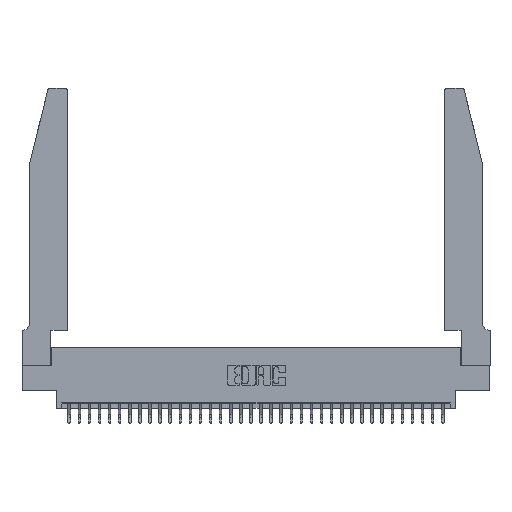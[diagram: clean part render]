
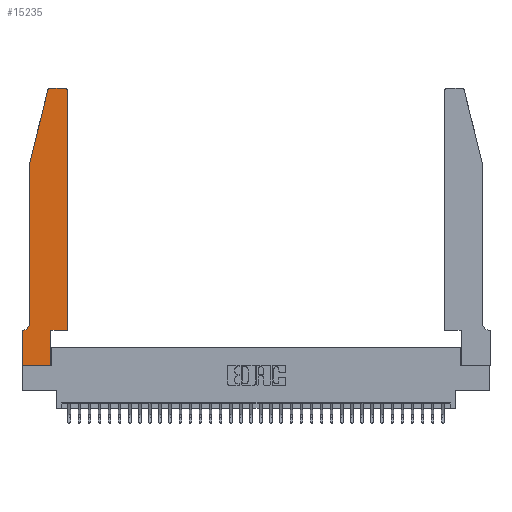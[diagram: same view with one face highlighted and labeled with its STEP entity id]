
A CAD part, top view. The second image highlights one B-rep face of the part: STEP entity #15235.
In plain terms, the highlighted planar face has unit normal (0, 0, 1).
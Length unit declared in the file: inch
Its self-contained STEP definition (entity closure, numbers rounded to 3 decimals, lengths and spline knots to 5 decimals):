
#98 = LINE ( 'NONE', #8439, #7492 ) ;
#121 = VECTOR ( 'NONE', #23977, 39.37008 ) ;
#1457 = CARTESIAN_POINT ( 'NONE',  ( 0.2865, 0.35, 0.37 ) ) ;
#1524 = AXIS2_PLACEMENT_3D ( 'NONE', #26962, #10634, #29683 ) ;
#1671 = VECTOR ( 'NONE', #10554, 39.37008 ) ;
#1958 = DIRECTION ( 'NONE',  ( 1., 0., 0. ) ) ;
#2000 = CARTESIAN_POINT ( 'NONE',  ( 0.0755, 2., 0.37 ) ) ;
#2250 = CARTESIAN_POINT ( 'NONE',  ( 0.0755, 2., 0.37 ) ) ;
#2755 = EDGE_CURVE ( 'NONE', #16288, #17330, #23582, .T. ) ;
#3211 = VECTOR ( 'NONE', #24135, 39.37008 ) ;
#3431 = EDGE_CURVE ( 'NONE', #17330, #6809, #3760, .T. ) ;
#3760 = CIRCLE ( 'NONE', #1524, 0.03 ) ;
#4895 = CARTESIAN_POINT ( 'NONE',  ( 0., 0., 0.37 ) ) ;
#5574 = EDGE_CURVE ( 'NONE', #13917, #17988, #11427, .T. ) ;
#5582 = ORIENTED_EDGE ( 'NONE', *, *, #17892, .T. ) ;
#5916 = AXIS2_PLACEMENT_3D ( 'NONE', #6968, #26132, #9776 ) ;
#6114 = VERTEX_POINT ( 'NONE', #1457 ) ;
#6215 = CARTESIAN_POINT ( 'NONE',  ( 0.2865, 0., 0.37 ) ) ;
#6584 = VECTOR ( 'NONE', #7798, 39.37008 ) ;
#6809 = VERTEX_POINT ( 'NONE', #15743 ) ;
#6968 = CARTESIAN_POINT ( 'NONE',  ( 0., 0.35, 0.37 ) ) ;
#7492 = VECTOR ( 'NONE', #16575, 39.37008 ) ;
#7798 = DIRECTION ( 'NONE',  ( 0., 1., 0. ) ) ;
#8439 = CARTESIAN_POINT ( 'NONE',  ( 0.4505, 0.35, 0.37 ) ) ;
#9776 = DIRECTION ( 'NONE',  ( 1., 0., 0. ) ) ;
#10435 = CARTESIAN_POINT ( 'NONE',  ( 0.0755, 0.35, 0.37 ) ) ;
#10516 = CARTESIAN_POINT ( 'NONE',  ( 0.0755, 0.42, 0.37 ) ) ;
#10554 = DIRECTION ( 'NONE',  ( 0., 1., 0. ) ) ;
#10634 = DIRECTION ( 'NONE',  ( 0., 0., 1. ) ) ;
#11224 = CARTESIAN_POINT ( 'NONE',  ( 0.0055, 0.35, 0.37 ) ) ;
#11427 = CIRCLE ( 'NONE', #34774, 0.03 ) ;
#12835 = LINE ( 'NONE', #4895, #13697 ) ;
#12879 = VECTOR ( 'NONE', #24239, 39.37008 ) ;
#13174 = DIRECTION ( 'NONE',  ( -1., 0., 0. ) ) ;
#13500 = EDGE_CURVE ( 'NONE', #28595, #25222, #12835, .T. ) ;
#13697 = VECTOR ( 'NONE', #21323, 39.37008 ) ;
#13917 = VERTEX_POINT ( 'NONE', #25642 ) ;
#14008 = CARTESIAN_POINT ( 'NONE',  ( 0.0055, 0.42, 0.37 ) ) ;
#14090 = CARTESIAN_POINT ( 'NONE',  ( 0.2605, 2.75, 0.37 ) ) ;
#14626 = ORIENTED_EDGE ( 'NONE', *, *, #21843, .T. ) ;
#14770 = EDGE_CURVE ( 'NONE', #20298, #28595, #19566, .T. ) ;
#15235 = ADVANCED_FACE ( 'NONE', ( #22509 ), #23388, .T. ) ;
#15743 = CARTESIAN_POINT ( 'NONE',  ( 0.4205, 2.75, 0.37 ) ) ;
#16288 = VERTEX_POINT ( 'NONE', #28972 ) ;
#16458 = EDGE_CURVE ( 'NONE', #25222, #6114, #27547, .T. ) ;
#16575 = DIRECTION ( 'NONE',  ( 1., 0., 0. ) ) ;
#16735 = DIRECTION ( 'NONE',  ( -1., 0., 0. ) ) ;
#16807 = ORIENTED_EDGE ( 'NONE', *, *, #2755, .T. ) ;
#17101 = CARTESIAN_POINT ( 'NONE',  ( 0.4505, 2.72, 0.37 ) ) ;
#17330 = VERTEX_POINT ( 'NONE', #17101 ) ;
#17892 = EDGE_CURVE ( 'NONE', #6114, #16288, #98, .T. ) ;
#17988 = VERTEX_POINT ( 'NONE', #28047 ) ;
#18004 = LINE ( 'NONE', #10435, #31654 ) ;
#18415 = DIRECTION ( 'NONE',  ( 0., 0., 1. ) ) ;
#18710 = ORIENTED_EDGE ( 'NONE', *, *, #26153, .T. ) ;
#19566 = LINE ( 'NONE', #32288, #3211 ) ;
#20298 = VERTEX_POINT ( 'NONE', #27846 ) ;
#20536 = VECTOR ( 'NONE', #30383, 39.37008 ) ;
#20577 = ORIENTED_EDGE ( 'NONE', *, *, #16458, .T. ) ;
#21101 = ORIENTED_EDGE ( 'NONE', *, *, #3431, .T. ) ;
#21177 = CARTESIAN_POINT ( 'NONE',  ( 0., 0., 0.37 ) ) ;
#21323 = DIRECTION ( 'NONE',  ( 1., 0., 0. ) ) ;
#21843 = EDGE_CURVE ( 'NONE', #29856, #33451, #22706, .T. ) ;
#22509 = FACE_OUTER_BOUND ( 'NONE', #23521, .T. ) ;
#22706 = CIRCLE ( 'NONE', #31878, 0.07 ) ;
#23388 = PLANE ( 'NONE',  #5916 ) ;
#23521 = EDGE_LOOP ( 'NONE', ( #33191, #26815, #18710, #29000, #14626, #33312, #31191, #26534, #20577, #5582, #16807, #21101 ) ) ;
#23582 = LINE ( 'NONE', #29616, #1671 ) ;
#23977 = DIRECTION ( 'NONE',  ( -0.239, -0.971, 0. ) ) ;
#24135 = DIRECTION ( 'NONE',  ( 0., -1., 0. ) ) ;
#24214 = CARTESIAN_POINT ( 'NONE',  ( 0.2865, 0.35, 0.37 ) ) ;
#24239 = DIRECTION ( 'NONE',  ( 0., -1., 0. ) ) ;
#25222 = VERTEX_POINT ( 'NONE', #6215 ) ;
#25642 = CARTESIAN_POINT ( 'NONE',  ( 0.284, 2.75, 0.37 ) ) ;
#26132 = DIRECTION ( 'NONE',  ( 0., 0., 1. ) ) ;
#26153 = EDGE_CURVE ( 'NONE', #17988, #35333, #28500, .T. ) ;
#26534 = ORIENTED_EDGE ( 'NONE', *, *, #13500, .T. ) ;
#26815 = ORIENTED_EDGE ( 'NONE', *, *, #5574, .T. ) ;
#26962 = CARTESIAN_POINT ( 'NONE',  ( 0.4205, 2.72, 0.37 ) ) ;
#27547 = LINE ( 'NONE', #24214, #6584 ) ;
#27846 = CARTESIAN_POINT ( 'NONE',  ( 0., 0.35, 0.37 ) ) ;
#28047 = CARTESIAN_POINT ( 'NONE',  ( 0.25487, 2.72718, 0.37 ) ) ;
#28500 = LINE ( 'NONE', #2000, #121 ) ;
#28595 = VERTEX_POINT ( 'NONE', #21177 ) ;
#28972 = CARTESIAN_POINT ( 'NONE',  ( 0.4505, 0.35, 0.37 ) ) ;
#29000 = ORIENTED_EDGE ( 'NONE', *, *, #35063, .T. ) ;
#29616 = CARTESIAN_POINT ( 'NONE',  ( 0.4505, 0.35, 0.37 ) ) ;
#29683 = DIRECTION ( 'NONE',  ( 1., 0., 0. ) ) ;
#29856 = VERTEX_POINT ( 'NONE', #10516 ) ;
#30383 = DIRECTION ( 'NONE',  ( -1., 0., 0. ) ) ;
#31191 = ORIENTED_EDGE ( 'NONE', *, *, #14770, .T. ) ;
#31654 = VECTOR ( 'NONE', #13174, 39.37008 ) ;
#31878 = AXIS2_PLACEMENT_3D ( 'NONE', #14008, #33040, #16735 ) ;
#32288 = CARTESIAN_POINT ( 'NONE',  ( 0., 0., 0.37 ) ) ;
#33040 = DIRECTION ( 'NONE',  ( 0., 0., -1. ) ) ;
#33191 = ORIENTED_EDGE ( 'NONE', *, *, #35268, .T. ) ;
#33312 = ORIENTED_EDGE ( 'NONE', *, *, #34478, .T. ) ;
#33354 = CARTESIAN_POINT ( 'NONE',  ( 0.0755, 2., 0.37 ) ) ;
#33451 = VERTEX_POINT ( 'NONE', #11224 ) ;
#34478 = EDGE_CURVE ( 'NONE', #33451, #20298, #18004, .T. ) ;
#34723 = CARTESIAN_POINT ( 'NONE',  ( 0.284, 2.72, 0.37 ) ) ;
#34774 = AXIS2_PLACEMENT_3D ( 'NONE', #34723, #18415, #1958 ) ;
#34987 = LINE ( 'NONE', #14090, #20536 ) ;
#35063 = EDGE_CURVE ( 'NONE', #35333, #29856, #35434, .T. ) ;
#35268 = EDGE_CURVE ( 'NONE', #6809, #13917, #34987, .T. ) ;
#35333 = VERTEX_POINT ( 'NONE', #33354 ) ;
#35434 = LINE ( 'NONE', #2250, #12879 ) ;
